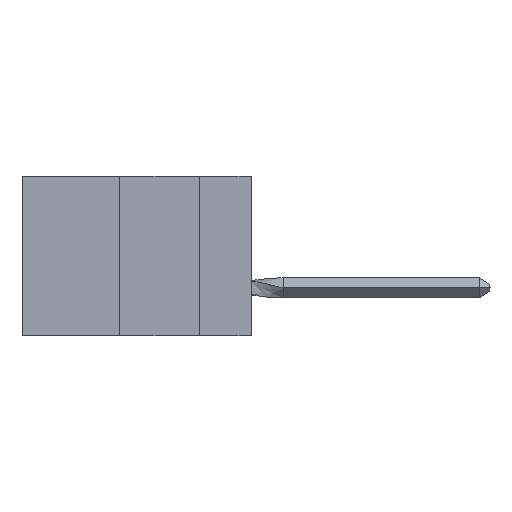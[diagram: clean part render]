
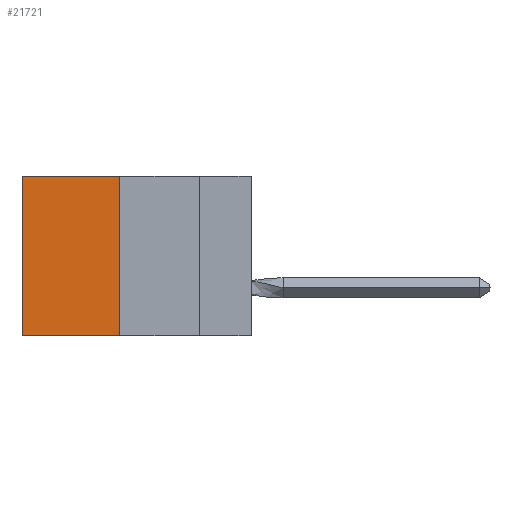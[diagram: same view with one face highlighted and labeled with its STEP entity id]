
A CAD part, left-side view. The second image highlights one B-rep face of the part: STEP entity #21721.
In plain terms, the highlighted planar face has unit normal (-1, 0, 0).
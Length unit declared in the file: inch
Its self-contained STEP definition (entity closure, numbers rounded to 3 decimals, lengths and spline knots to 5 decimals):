
#505 = VECTOR ( 'NONE', #2421, 39.37008 ) ;
#977 = EDGE_CURVE ( 'NONE', #23570, #3514, #16113, .T. ) ;
#2050 = EDGE_CURVE ( 'NONE', #13493, #23570, #28382, .T. ) ;
#2105 = CARTESIAN_POINT ( 'NONE',  ( 0.305, 0.413, 0. ) ) ;
#2279 = VECTOR ( 'NONE', #22782, 39.37008 ) ;
#2421 = DIRECTION ( 'NONE',  ( 0., 0., -1. ) ) ;
#2665 = PLANE ( 'NONE',  #26231 ) ;
#2898 = DIRECTION ( 'NONE',  ( 0., 0., -1. ) ) ;
#3514 = VERTEX_POINT ( 'NONE', #12278 ) ;
#3706 = ORIENTED_EDGE ( 'NONE', *, *, #2050, .T. ) ;
#4368 = CARTESIAN_POINT ( 'NONE',  ( 0.305, 0.413, -0.5 ) ) ;
#5435 = CARTESIAN_POINT ( 'NONE',  ( 0.305, 0.413, -0.5 ) ) ;
#6304 = VECTOR ( 'NONE', #2898, 39.37008 ) ;
#8208 = ORIENTED_EDGE ( 'NONE', *, *, #24844, .F. ) ;
#8650 = LINE ( 'NONE', #5435, #505 ) ;
#12156 = CARTESIAN_POINT ( 'NONE',  ( 0.305, 0.413, 0. ) ) ;
#12278 = CARTESIAN_POINT ( 'NONE',  ( 0.305, 0.72, -0.5 ) ) ;
#13493 = VERTEX_POINT ( 'NONE', #2105 ) ;
#15002 = DIRECTION ( 'NONE',  ( 0., 1., 0. ) ) ;
#16113 = LINE ( 'NONE', #24322, #6304 ) ;
#16838 = ORIENTED_EDGE ( 'NONE', *, *, #29748, .F. ) ;
#19747 = VERTEX_POINT ( 'NONE', #4368 ) ;
#19952 = CARTESIAN_POINT ( 'NONE',  ( 0.305, 0.413, -0.5 ) ) ;
#21721 = ADVANCED_FACE ( 'NONE', ( #30012 ), #2665, .F. ) ;
#21963 = VECTOR ( 'NONE', #15002, 39.37008 ) ;
#22782 = DIRECTION ( 'NONE',  ( 0., 1., 0. ) ) ;
#23570 = VERTEX_POINT ( 'NONE', #27639 ) ;
#24322 = CARTESIAN_POINT ( 'NONE',  ( 0.305, 0.72, -0.5 ) ) ;
#24844 = EDGE_CURVE ( 'NONE', #13493, #19747, #8650, .T. ) ;
#25298 = LINE ( 'NONE', #19952, #2279 ) ;
#26231 = AXIS2_PLACEMENT_3D ( 'NONE', #30110, #27222, #32974 ) ;
#27222 = DIRECTION ( 'NONE',  ( 1., 0., 0. ) ) ;
#27317 = ORIENTED_EDGE ( 'NONE', *, *, #977, .T. ) ;
#27639 = CARTESIAN_POINT ( 'NONE',  ( 0.305, 0.72, 0. ) ) ;
#28382 = LINE ( 'NONE', #12156, #21963 ) ;
#29748 = EDGE_CURVE ( 'NONE', #19747, #3514, #25298, .T. ) ;
#30012 = FACE_OUTER_BOUND ( 'NONE', #32738, .T. ) ;
#30110 = CARTESIAN_POINT ( 'NONE',  ( 0.305, 0.413, -0.5 ) ) ;
#32738 = EDGE_LOOP ( 'NONE', ( #27317, #16838, #8208, #3706 ) ) ;
#32974 = DIRECTION ( 'NONE',  ( 0., 0., -1. ) ) ;
